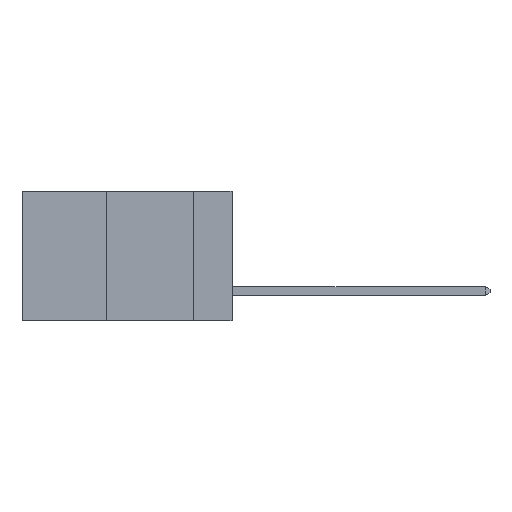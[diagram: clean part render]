
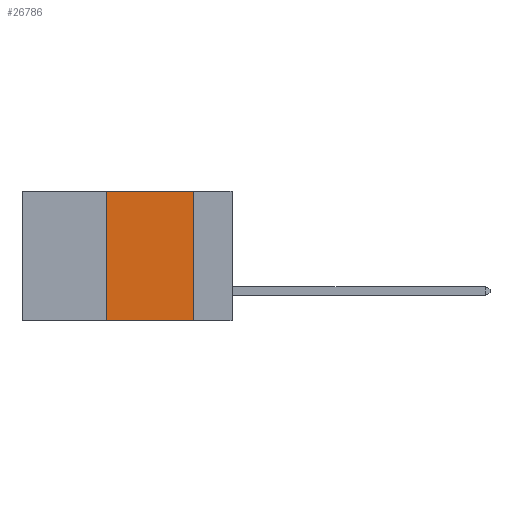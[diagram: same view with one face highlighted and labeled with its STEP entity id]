
A CAD part, left-side view. The second image highlights one B-rep face of the part: STEP entity #26786.
In plain terms, the highlighted planar face has unit normal (-1, 0, 0).
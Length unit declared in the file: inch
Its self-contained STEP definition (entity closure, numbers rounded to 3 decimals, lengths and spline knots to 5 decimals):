
#597 = VECTOR ( 'NONE', #1155, 39.37008 ) ;
#1155 = DIRECTION ( 'NONE',  ( 0., 0., 1. ) ) ;
#1192 = DIRECTION ( 'NONE',  ( 0., -1., 0. ) ) ;
#1254 = VERTEX_POINT ( 'NONE', #23007 ) ;
#1332 = ORIENTED_EDGE ( 'NONE', *, *, #25621, .F. ) ;
#2761 = VECTOR ( 'NONE', #27746, 39.37008 ) ;
#4787 = DIRECTION ( 'NONE',  ( 1., 0., 0. ) ) ;
#4845 = CARTESIAN_POINT ( 'NONE',  ( 0., 0.11, -0.37 ) ) ;
#7007 = CARTESIAN_POINT ( 'NONE',  ( 0., 0.36, 0. ) ) ;
#7363 = VERTEX_POINT ( 'NONE', #23633 ) ;
#9919 = CARTESIAN_POINT ( 'NONE',  ( 0., 0.11, 0. ) ) ;
#10290 = CARTESIAN_POINT ( 'NONE',  ( 0., 0.6, -0.37 ) ) ;
#10561 = PLANE ( 'NONE',  #28154 ) ;
#11489 = LINE ( 'NONE', #10290, #2761 ) ;
#11914 = ORIENTED_EDGE ( 'NONE', *, *, #13618, .T. ) ;
#13618 = EDGE_CURVE ( 'NONE', #1254, #27934, #11489, .T. ) ;
#16904 = EDGE_LOOP ( 'NONE', ( #1332, #16968, #17871, #11914 ) ) ;
#16968 = ORIENTED_EDGE ( 'NONE', *, *, #21218, .F. ) ;
#17064 = CARTESIAN_POINT ( 'NONE',  ( 0., 0.11, 0. ) ) ;
#17699 = VECTOR ( 'NONE', #31636, 39.37008 ) ;
#17871 = ORIENTED_EDGE ( 'NONE', *, *, #29945, .F. ) ;
#18617 = LINE ( 'NONE', #17064, #17699 ) ;
#19389 = CARTESIAN_POINT ( 'NONE',  ( 0., 0.6, 0. ) ) ;
#21218 = EDGE_CURVE ( 'NONE', #7363, #23457, #28027, .T. ) ;
#23007 = CARTESIAN_POINT ( 'NONE',  ( 0., 0.36, -0.37 ) ) ;
#23457 = VERTEX_POINT ( 'NONE', #9919 ) ;
#23633 = CARTESIAN_POINT ( 'NONE',  ( 0., 0.36, 0. ) ) ;
#24951 = LINE ( 'NONE', #7007, #597 ) ;
#25269 = DIRECTION ( 'NONE',  ( 0., 0., -1. ) ) ;
#25621 = EDGE_CURVE ( 'NONE', #23457, #27934, #18617, .T. ) ;
#26786 = ADVANCED_FACE ( 'NONE', ( #35060 ), #10561, .F. ) ;
#27746 = DIRECTION ( 'NONE',  ( 0., -1., 0. ) ) ;
#27934 = VERTEX_POINT ( 'NONE', #4845 ) ;
#28027 = LINE ( 'NONE', #30330, #34766 ) ;
#28154 = AXIS2_PLACEMENT_3D ( 'NONE', #19389, #4787, #25269 ) ;
#29945 = EDGE_CURVE ( 'NONE', #1254, #7363, #24951, .T. ) ;
#30330 = CARTESIAN_POINT ( 'NONE',  ( 0., 0.6, 0. ) ) ;
#31636 = DIRECTION ( 'NONE',  ( 0., 0., -1. ) ) ;
#34766 = VECTOR ( 'NONE', #1192, 39.37008 ) ;
#35060 = FACE_OUTER_BOUND ( 'NONE', #16904, .T. ) ;
